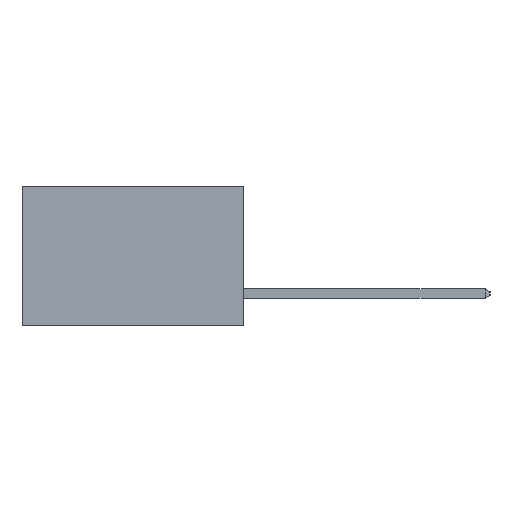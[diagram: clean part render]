
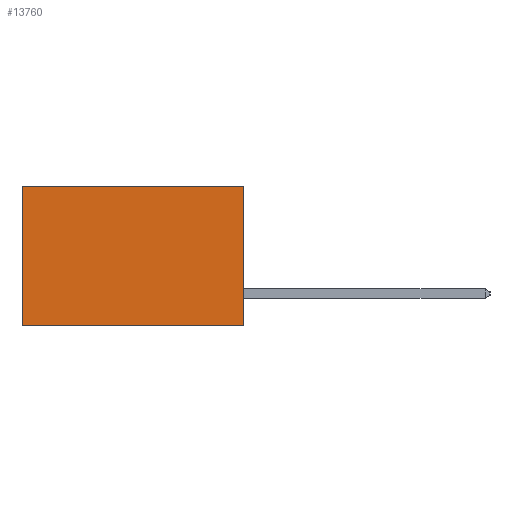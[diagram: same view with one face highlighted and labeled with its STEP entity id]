
A CAD part, left-side view. The second image highlights one B-rep face of the part: STEP entity #13760.
In plain terms, the highlighted planar face has unit normal (-1, 0, 0).
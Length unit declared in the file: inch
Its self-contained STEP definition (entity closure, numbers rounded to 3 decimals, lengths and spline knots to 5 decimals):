
#92 = CARTESIAN_POINT ( 'NONE',  ( 0.277, 0., 0. ) ) ;
#561 = DIRECTION ( 'NONE',  ( 0., 1., 0. ) ) ;
#997 = LINE ( 'NONE', #11441, #5046 ) ;
#1567 = EDGE_CURVE ( 'NONE', #19873, #14671, #20485, .T. ) ;
#2135 = CARTESIAN_POINT ( 'NONE',  ( 0.277, 0., -0.37 ) ) ;
#4374 = LINE ( 'NONE', #16451, #8347 ) ;
#5046 = VECTOR ( 'NONE', #18183, 39.37008 ) ;
#5279 = CARTESIAN_POINT ( 'NONE',  ( 0.277, 0., -0.37 ) ) ;
#5591 = DIRECTION ( 'NONE',  ( 0., 0., -1. ) ) ;
#6020 = ORIENTED_EDGE ( 'NONE', *, *, #14774, .T. ) ;
#6510 = VECTOR ( 'NONE', #561, 39.37008 ) ;
#8347 = VECTOR ( 'NONE', #11470, 39.37008 ) ;
#10137 = ORIENTED_EDGE ( 'NONE', *, *, #12195, .F. ) ;
#11441 = CARTESIAN_POINT ( 'NONE',  ( 0.277, 0., -0.37 ) ) ;
#11470 = DIRECTION ( 'NONE',  ( 0., 0., -1. ) ) ;
#12195 = EDGE_CURVE ( 'NONE', #19873, #17536, #997, .T. ) ;
#12646 = ORIENTED_EDGE ( 'NONE', *, *, #1567, .T. ) ;
#12930 = DIRECTION ( 'NONE',  ( 0., 1., 0. ) ) ;
#13760 = ADVANCED_FACE ( 'NONE', ( #20520 ), #18997, .F. ) ;
#14268 = CARTESIAN_POINT ( 'NONE',  ( 0.277, 0., 0. ) ) ;
#14671 = VERTEX_POINT ( 'NONE', #17936 ) ;
#14774 = EDGE_CURVE ( 'NONE', #14671, #19457, #4374, .T. ) ;
#15575 = VECTOR ( 'NONE', #12930, 39.37008 ) ;
#15714 = DIRECTION ( 'NONE',  ( 1., 0., 0. ) ) ;
#16451 = CARTESIAN_POINT ( 'NONE',  ( 0.277, 0.59, -0.37 ) ) ;
#16708 = ORIENTED_EDGE ( 'NONE', *, *, #18639, .F. ) ;
#17536 = VERTEX_POINT ( 'NONE', #5279 ) ;
#17936 = CARTESIAN_POINT ( 'NONE',  ( 0.277, 0.59, 0. ) ) ;
#18183 = DIRECTION ( 'NONE',  ( 0., 0., -1. ) ) ;
#18520 = EDGE_LOOP ( 'NONE', ( #6020, #16708, #10137, #12646 ) ) ;
#18639 = EDGE_CURVE ( 'NONE', #17536, #19457, #20534, .T. ) ;
#18997 = PLANE ( 'NONE',  #21885 ) ;
#19457 = VERTEX_POINT ( 'NONE', #19978 ) ;
#19580 = CARTESIAN_POINT ( 'NONE',  ( 0.277, 0., -0.37 ) ) ;
#19873 = VERTEX_POINT ( 'NONE', #14268 ) ;
#19978 = CARTESIAN_POINT ( 'NONE',  ( 0.277, 0.59, -0.37 ) ) ;
#20485 = LINE ( 'NONE', #92, #6510 ) ;
#20520 = FACE_OUTER_BOUND ( 'NONE', #18520, .T. ) ;
#20534 = LINE ( 'NONE', #19580, #15575 ) ;
#21885 = AXIS2_PLACEMENT_3D ( 'NONE', #2135, #15714, #5591 ) ;
